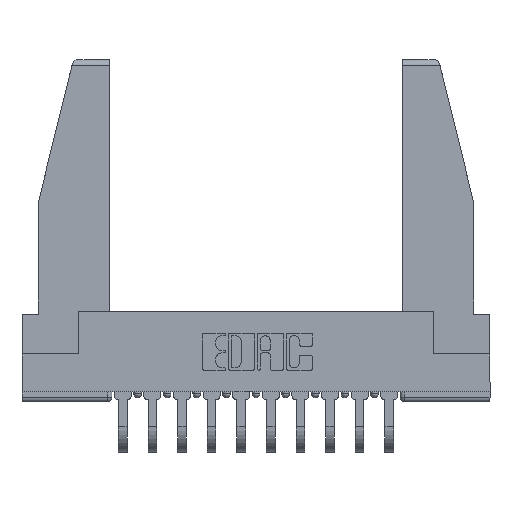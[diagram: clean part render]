
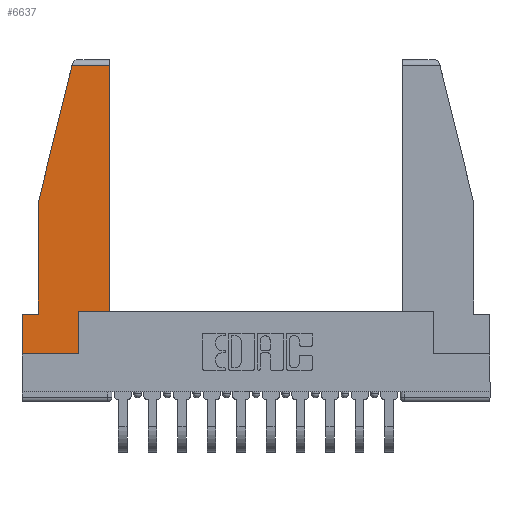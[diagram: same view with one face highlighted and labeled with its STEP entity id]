
A CAD part, top view. The second image highlights one B-rep face of the part: STEP entity #6637.
In plain terms, the highlighted planar face has unit normal (0, 0, 1).
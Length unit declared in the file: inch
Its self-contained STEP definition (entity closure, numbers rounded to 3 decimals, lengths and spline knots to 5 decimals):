
#59 = CARTESIAN_POINT ( 'NONE',  ( 0.271, 1.55, 0. ) ) ;
#61 = CARTESIAN_POINT ( 'NONE',  ( 0.461, 0.223, 0. ) ) ;
#149 = CARTESIAN_POINT ( 'NONE',  ( 0., 0.21, 0. ) ) ;
#493 = ORIENTED_EDGE ( 'NONE', *, *, #7875, .T. ) ;
#577 = PLANE ( 'NONE',  #6661 ) ;
#917 = CARTESIAN_POINT ( 'NONE',  ( 0.461, 0.223, 0. ) ) ;
#934 = DIRECTION ( 'NONE',  ( -1., 0., 0. ) ) ;
#992 = ORIENTED_EDGE ( 'NONE', *, *, #3226, .T. ) ;
#1317 = VERTEX_POINT ( 'NONE', #13287 ) ;
#1342 = CARTESIAN_POINT ( 'NONE',  ( 0.297, 0.223, 0. ) ) ;
#1421 = EDGE_CURVE ( 'NONE', #11646, #12728, #11819, .T. ) ;
#1891 = CARTESIAN_POINT ( 'NONE',  ( 0.297, 0.223, 0. ) ) ;
#2252 = VECTOR ( 'NONE', #12658, 39.37008 ) ;
#2510 = DIRECTION ( 'NONE',  ( -1., 0., 0. ) ) ;
#2511 = CARTESIAN_POINT ( 'NONE',  ( 0.2636, 1.52, 0. ) ) ;
#2787 = VECTOR ( 'NONE', #4711, 39.37008 ) ;
#2842 = LINE ( 'NONE', #14521, #12123 ) ;
#2989 = CARTESIAN_POINT ( 'NONE',  ( 0.461, 1.52, 0. ) ) ;
#3103 = VERTEX_POINT ( 'NONE', #14223 ) ;
#3121 = ORIENTED_EDGE ( 'NONE', *, *, #1421, .T. ) ;
#3226 = EDGE_CURVE ( 'NONE', #13720, #5683, #14297, .T. ) ;
#3395 = LINE ( 'NONE', #7811, #5580 ) ;
#3492 = VECTOR ( 'NONE', #2510, 39.37008 ) ;
#3736 = ORIENTED_EDGE ( 'NONE', *, *, #3849, .T. ) ;
#3849 = EDGE_CURVE ( 'NONE', #15090, #3103, #13444, .T. ) ;
#3915 = DIRECTION ( 'NONE',  ( 1., 0., 0. ) ) ;
#3944 = DIRECTION ( 'NONE',  ( 0., 1., 0. ) ) ;
#4055 = DIRECTION ( 'NONE',  ( 0., -1., 0. ) ) ;
#4349 = EDGE_LOOP ( 'NONE', ( #493, #5172, #14462, #11299, #3736, #7125, #992, #7372, #3121 ) ) ;
#4514 = VECTOR ( 'NONE', #3915, 39.37008 ) ;
#4711 = DIRECTION ( 'NONE',  ( 0., 1., 0. ) ) ;
#5172 = ORIENTED_EDGE ( 'NONE', *, *, #12257, .T. ) ;
#5222 = CARTESIAN_POINT ( 'NONE',  ( 0.086, 0.21, 0. ) ) ;
#5232 = LINE ( 'NONE', #14402, #13109 ) ;
#5237 = DIRECTION ( 'NONE',  ( 1., 0., 0. ) ) ;
#5580 = VECTOR ( 'NONE', #12715, 39.37008 ) ;
#5683 = VERTEX_POINT ( 'NONE', #11912 ) ;
#5927 = EDGE_CURVE ( 'NONE', #7616, #1317, #9275, .T. ) ;
#6197 = CARTESIAN_POINT ( 'NONE',  ( 0., 0., 0. ) ) ;
#6256 = VECTOR ( 'NONE', #934, 39.37008 ) ;
#6637 = ADVANCED_FACE ( 'NONE', ( #11269 ), #577, .T. ) ;
#6661 = AXIS2_PLACEMENT_3D ( 'NONE', #12501, #12349, #5237 ) ;
#7125 = ORIENTED_EDGE ( 'NONE', *, *, #13977, .T. ) ;
#7279 = CARTESIAN_POINT ( 'NONE',  ( 0., 0., 0. ) ) ;
#7372 = ORIENTED_EDGE ( 'NONE', *, *, #12116, .T. ) ;
#7510 = VECTOR ( 'NONE', #11673, 39.37008 ) ;
#7616 = VERTEX_POINT ( 'NONE', #2511 ) ;
#7811 = CARTESIAN_POINT ( 'NONE',  ( 0., 0.21, 0. ) ) ;
#7875 = EDGE_CURVE ( 'NONE', #12728, #11221, #10507, .T. ) ;
#9275 = LINE ( 'NONE', #59, #2252 ) ;
#9404 = LINE ( 'NONE', #14084, #6256 ) ;
#10444 = EDGE_CURVE ( 'NONE', #1317, #15090, #2842, .T. ) ;
#10507 = LINE ( 'NONE', #61, #2787 ) ;
#11221 = VERTEX_POINT ( 'NONE', #2989 ) ;
#11269 = FACE_OUTER_BOUND ( 'NONE', #4349, .T. ) ;
#11299 = ORIENTED_EDGE ( 'NONE', *, *, #10444, .T. ) ;
#11646 = VERTEX_POINT ( 'NONE', #1891 ) ;
#11673 = DIRECTION ( 'NONE',  ( 1., 0., 0. ) ) ;
#11819 = LINE ( 'NONE', #1342, #7510 ) ;
#11912 = CARTESIAN_POINT ( 'NONE',  ( 0.297, 0., 0. ) ) ;
#12116 = EDGE_CURVE ( 'NONE', #5683, #11646, #5232, .T. ) ;
#12123 = VECTOR ( 'NONE', #4055, 39.37008 ) ;
#12257 = EDGE_CURVE ( 'NONE', #11221, #7616, #9404, .T. ) ;
#12349 = DIRECTION ( 'NONE',  ( 0., 0., 1. ) ) ;
#12501 = CARTESIAN_POINT ( 'NONE',  ( 0., 0., 0. ) ) ;
#12658 = DIRECTION ( 'NONE',  ( -0.239, -0.971, 0. ) ) ;
#12715 = DIRECTION ( 'NONE',  ( 0., -1., 0. ) ) ;
#12728 = VERTEX_POINT ( 'NONE', #917 ) ;
#13109 = VECTOR ( 'NONE', #3944, 39.37008 ) ;
#13287 = CARTESIAN_POINT ( 'NONE',  ( 0.086, 0.8, 0. ) ) ;
#13444 = LINE ( 'NONE', #149, #3492 ) ;
#13720 = VERTEX_POINT ( 'NONE', #7279 ) ;
#13977 = EDGE_CURVE ( 'NONE', #3103, #13720, #3395, .T. ) ;
#14084 = CARTESIAN_POINT ( 'NONE',  ( 0., 1.52, 0. ) ) ;
#14223 = CARTESIAN_POINT ( 'NONE',  ( 0., 0.21, 0. ) ) ;
#14297 = LINE ( 'NONE', #6197, #4514 ) ;
#14402 = CARTESIAN_POINT ( 'NONE',  ( 0.297, 0., 0. ) ) ;
#14462 = ORIENTED_EDGE ( 'NONE', *, *, #5927, .T. ) ;
#14521 = CARTESIAN_POINT ( 'NONE',  ( 0.086, 0.8, 0. ) ) ;
#15090 = VERTEX_POINT ( 'NONE', #5222 ) ;
